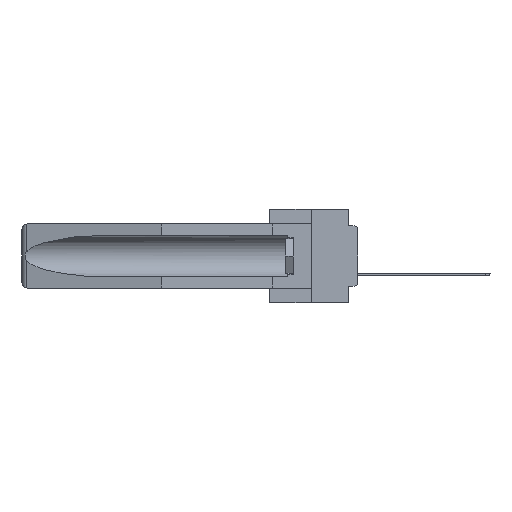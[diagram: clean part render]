
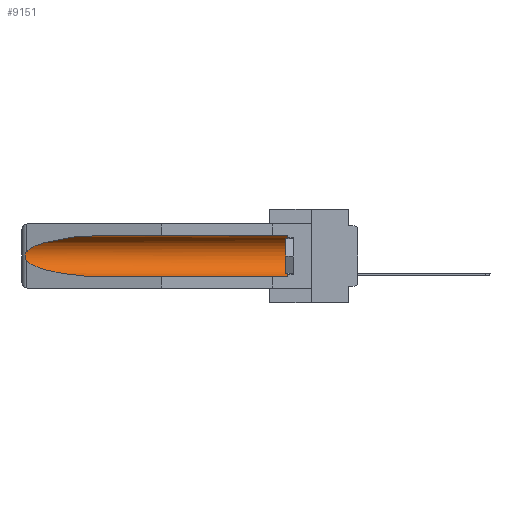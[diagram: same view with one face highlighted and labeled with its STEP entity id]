
A CAD part, left-side view. The second image highlights one B-rep face of the part: STEP entity #9151.
In plain terms, the highlighted cylindrical face has radius 2.857 mm (diameter 5.715 mm), a partial arc.
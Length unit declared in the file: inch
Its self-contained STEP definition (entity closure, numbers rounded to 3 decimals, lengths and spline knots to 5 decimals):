
#117 = EDGE_CURVE ( 'NONE', #8384, #30590, #22216, .T. ) ;
#1194 = CARTESIAN_POINT ( 'NONE',  ( 0.155, 1.07973, -0.284 ) ) ;
#1567 = ORIENTED_EDGE ( 'NONE', *, *, #117, .T. ) ;
#1784 = CARTESIAN_POINT ( 'NONE',  ( 0.26597, 1.5296, -0.19026 ) ) ;
#2367 = CARTESIAN_POINT ( 'NONE',  ( 0.26537, 1.52718, -0.19328 ) ) ;
#3108 = DIRECTION ( 'NONE',  ( 0., 0., 1. ) ) ;
#3449 = CARTESIAN_POINT ( 'NONE',  ( 0.155, 0.126, -0.1715 ) ) ;
#3530 = VERTEX_POINT ( 'NONE', #31132 ) ;
#3703 = EDGE_LOOP ( 'NONE', ( #17868, #8611, #1567, #34778, #15285, #33924 ) ) ;
#4236 = VECTOR ( 'NONE', #25073, 39.37008 ) ;
#5228 = VERTEX_POINT ( 'NONE', #19135 ) ;
#5387 = CARTESIAN_POINT ( 'NONE',  ( 0.21114, 1.30732, -0.284 ) ) ;
#5755 = VERTEX_POINT ( 'NONE', #13749 ) ;
#5829 = LINE ( 'NONE', #25076, #4236 ) ;
#5872 = DIRECTION ( 'NONE',  ( 0., 1., 0. ) ) ;
#7851 = CARTESIAN_POINT ( 'NONE',  ( 0.2673, 1.5327, -0.16383 ) ) ;
#8384 = VERTEX_POINT ( 'NONE', #2367 ) ;
#8557 = VERTEX_POINT ( 'NONE', #35265 ) ;
#8611 = ORIENTED_EDGE ( 'NONE', *, *, #16815, .T. ) ;
#8705 = EDGE_CURVE ( 'NONE', #5228, #5755, #28579, .T. ) ;
#9072 = CARTESIAN_POINT ( 'NONE',  ( 0.25451, 1.48313, -0.09465 ) ) ;
#9151 = ADVANCED_FACE ( 'NONE', ( #33728 ), #19804, .F. ) ;
#9507 = EDGE_CURVE ( 'NONE', #5228, #30590, #5829, .T. ) ;
#10218 = CARTESIAN_POINT ( 'NONE',  ( 0.26597, 1.52961, -0.15275 ) ) ;
#11812 = AXIS2_PLACEMENT_3D ( 'NONE', #30994, #5872, #3108 ) ;
#13749 = CARTESIAN_POINT ( 'NONE',  ( 0.155, 0.126, -0.059 ) ) ;
#13802 = VECTOR ( 'NONE', #32484, 39.37008 ) ;
#14621 = DIRECTION ( 'NONE',  ( 0., -1., 0. ) ) ;
#15285 = ORIENTED_EDGE ( 'NONE', *, *, #8705, .T. ) ;
#16081 = CARTESIAN_POINT ( 'NONE',  ( 0.2673, 1.53269, -0.17917 ) ) ;
#16815 = EDGE_CURVE ( 'NONE', #3530, #8384, #25500, .T. ) ;
#17868 = ORIENTED_EDGE ( 'NONE', *, *, #21538, .T. ) ;
#18658 = AXIS2_PLACEMENT_3D ( 'NONE', #3449, #14621, #31496 ) ;
#18662 = CARTESIAN_POINT ( 'NONE',  ( 0.26655, 1.53094, -0.18657 ) ) ;
#19135 = CARTESIAN_POINT ( 'NONE',  ( 0.155, 0.126, -0.284 ) ) ;
#19316 = CARTESIAN_POINT ( 'NONE',  ( 0.26537, 1.52718, -0.19328 ) ) ;
#19804 = CYLINDRICAL_SURFACE ( 'NONE', #11812, 0.1125 ) ;
#21538 = EDGE_CURVE ( 'NONE', #8557, #3530, #24577, .T. ) ;
#21665 = LINE ( 'NONE', #32843, #13802 ) ;
#22216 =( BOUNDED_CURVE ( )  B_SPLINE_CURVE ( 3, ( #19316, #30493, #5387, #36167 ),
 .UNSPECIFIED., .F., .T. ) 
 B_SPLINE_CURVE_WITH_KNOTS ( ( 4, 4 ),
 ( 0.1948, 1.5708 ),
 .UNSPECIFIED. ) 
 CURVE ( )  GEOMETRIC_REPRESENTATION_ITEM ( )  RATIONAL_B_SPLINE_CURVE ( ( 1., 0.848, 0.848, 1. ) ) 
 REPRESENTATION_ITEM ( '' )  );
#22272 = CARTESIAN_POINT ( 'NONE',  ( 0.155, 1.07973, -0.059 ) ) ;
#22995 = CARTESIAN_POINT ( 'NONE',  ( 0.21114, 1.30732, -0.059 ) ) ;
#24577 =( BOUNDED_CURVE ( )  B_SPLINE_CURVE ( 3, ( #22272, #22995, #9072, #33456 ),
 .UNSPECIFIED., .F., .T. ) 
 B_SPLINE_CURVE_WITH_KNOTS ( ( 4, 4 ),
 ( 4.71239, 6.08839 ),
 .UNSPECIFIED. ) 
 CURVE ( )  GEOMETRIC_REPRESENTATION_ITEM ( )  RATIONAL_B_SPLINE_CURVE ( ( 1., 0.848, 0.848, 1. ) ) 
 REPRESENTATION_ITEM ( '' )  );
#25073 = DIRECTION ( 'NONE',  ( 0., 1., 0. ) ) ;
#25076 = CARTESIAN_POINT ( 'NONE',  ( 0.155, -0.30754, -0.284 ) ) ;
#25500 = B_SPLINE_CURVE_WITH_KNOTS ( 'NONE', 3,
 ( #32417, #10218, #30391, #7851, #33140, #35506, #16081, #18662, #1784, #27252 ),
 .UNSPECIFIED., .F., .F.,
 ( 4, 2, 2, 2, 4 ),
 ( 0., 0.00029, 0.00058, 0.00087, 0.00117 ),
 .UNSPECIFIED. ) ;
#25873 = EDGE_CURVE ( 'NONE', #5755, #8557, #21665, .T. ) ;
#27252 = CARTESIAN_POINT ( 'NONE',  ( 0.26537, 1.52718, -0.19328 ) ) ;
#28579 = CIRCLE ( 'NONE', #18658, 0.1125 ) ;
#30391 = CARTESIAN_POINT ( 'NONE',  ( 0.26654, 1.53092, -0.15636 ) ) ;
#30493 = CARTESIAN_POINT ( 'NONE',  ( 0.25451, 1.48313, -0.24835 ) ) ;
#30590 = VERTEX_POINT ( 'NONE', #1194 ) ;
#30994 = CARTESIAN_POINT ( 'NONE',  ( 0.155, -0.30754, -0.1715 ) ) ;
#31132 = CARTESIAN_POINT ( 'NONE',  ( 0.26537, 1.52718, -0.14972 ) ) ;
#31496 = DIRECTION ( 'NONE',  ( 0., 0., 1. ) ) ;
#32417 = CARTESIAN_POINT ( 'NONE',  ( 0.26537, 1.52718, -0.14972 ) ) ;
#32484 = DIRECTION ( 'NONE',  ( 0., 1., 0. ) ) ;
#32843 = CARTESIAN_POINT ( 'NONE',  ( 0.155, -0.30754, -0.059 ) ) ;
#33140 = CARTESIAN_POINT ( 'NONE',  ( 0.2675, 1.53308, -0.16763 ) ) ;
#33456 = CARTESIAN_POINT ( 'NONE',  ( 0.26537, 1.52718, -0.14972 ) ) ;
#33728 = FACE_OUTER_BOUND ( 'NONE', #3703, .T. ) ;
#33924 = ORIENTED_EDGE ( 'NONE', *, *, #25873, .T. ) ;
#34778 = ORIENTED_EDGE ( 'NONE', *, *, #9507, .F. ) ;
#35265 = CARTESIAN_POINT ( 'NONE',  ( 0.155, 1.07973, -0.059 ) ) ;
#35506 = CARTESIAN_POINT ( 'NONE',  ( 0.2675, 1.53308, -0.17534 ) ) ;
#36167 = CARTESIAN_POINT ( 'NONE',  ( 0.155, 1.07973, -0.284 ) ) ;
